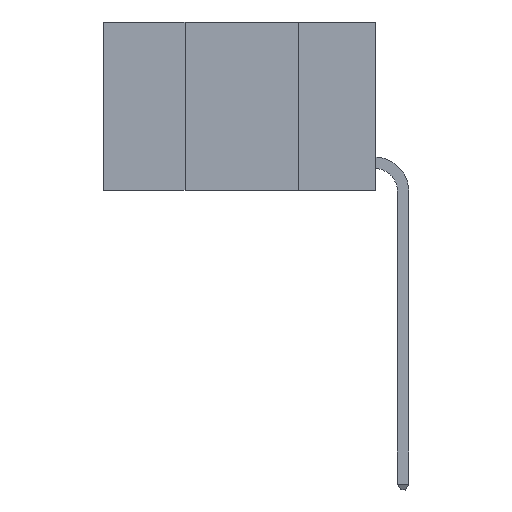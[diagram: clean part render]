
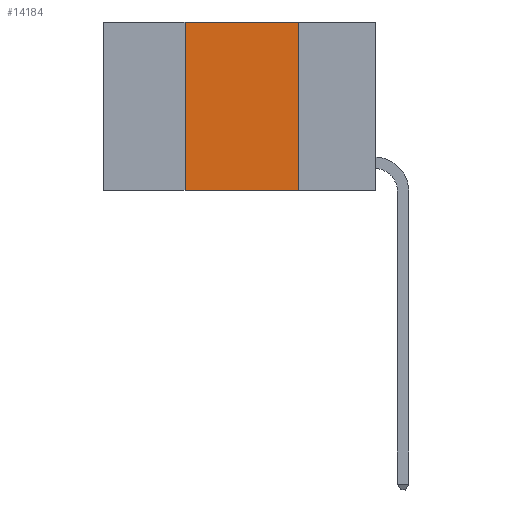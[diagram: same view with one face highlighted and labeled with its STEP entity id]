
A CAD part, left-side view. The second image highlights one B-rep face of the part: STEP entity #14184.
In plain terms, the highlighted planar face has unit normal (-1, 0, 0).
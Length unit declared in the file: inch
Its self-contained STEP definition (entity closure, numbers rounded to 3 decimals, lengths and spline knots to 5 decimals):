
#149 = CARTESIAN_POINT ( 'NONE',  ( 0., 0.17, -0.37 ) ) ;
#1687 = DIRECTION ( 'NONE',  ( 0., -1., 0. ) ) ;
#3434 = VERTEX_POINT ( 'NONE', #149 ) ;
#4382 = PLANE ( 'NONE',  #16585 ) ;
#5093 = EDGE_CURVE ( 'NONE', #20444, #3434, #11874, .T. ) ;
#5717 = LINE ( 'NONE', #27364, #12576 ) ;
#6720 = DIRECTION ( 'NONE',  ( 1., 0., 0. ) ) ;
#7209 = CARTESIAN_POINT ( 'NONE',  ( 0., 0.42, 0. ) ) ;
#8197 = EDGE_CURVE ( 'NONE', #22314, #3434, #5717, .T. ) ;
#8569 = EDGE_LOOP ( 'NONE', ( #14014, #21543, #13680, #11187 ) ) ;
#10779 = CARTESIAN_POINT ( 'NONE',  ( 0., 0.42, 0. ) ) ;
#11187 = ORIENTED_EDGE ( 'NONE', *, *, #5093, .T. ) ;
#11309 = FACE_OUTER_BOUND ( 'NONE', #8569, .T. ) ;
#11874 = LINE ( 'NONE', #22303, #29333 ) ;
#12576 = VECTOR ( 'NONE', #29629, 39.37008 ) ;
#12588 = CARTESIAN_POINT ( 'NONE',  ( 0., 0.42, -0.37 ) ) ;
#12648 = EDGE_CURVE ( 'NONE', #13353, #22314, #21616, .T. ) ;
#13353 = VERTEX_POINT ( 'NONE', #10779 ) ;
#13556 = CARTESIAN_POINT ( 'NONE',  ( 0., 0.6, 0. ) ) ;
#13680 = ORIENTED_EDGE ( 'NONE', *, *, #28636, .F. ) ;
#14014 = ORIENTED_EDGE ( 'NONE', *, *, #8197, .F. ) ;
#14184 = ADVANCED_FACE ( 'NONE', ( #11309 ), #4382, .F. ) ;
#15556 = VECTOR ( 'NONE', #26659, 39.37008 ) ;
#15734 = CARTESIAN_POINT ( 'NONE',  ( 0., 0.17, 0. ) ) ;
#16585 = AXIS2_PLACEMENT_3D ( 'NONE', #13556, #6720, #22734 ) ;
#20444 = VERTEX_POINT ( 'NONE', #12588 ) ;
#21543 = ORIENTED_EDGE ( 'NONE', *, *, #12648, .F. ) ;
#21616 = LINE ( 'NONE', #28844, #15556 ) ;
#22303 = CARTESIAN_POINT ( 'NONE',  ( 0., 0.6, -0.37 ) ) ;
#22314 = VERTEX_POINT ( 'NONE', #15734 ) ;
#22734 = DIRECTION ( 'NONE',  ( 0., 0., -1. ) ) ;
#25398 = DIRECTION ( 'NONE',  ( 0., 0., 1. ) ) ;
#26659 = DIRECTION ( 'NONE',  ( 0., -1., 0. ) ) ;
#27364 = CARTESIAN_POINT ( 'NONE',  ( 0., 0.17, 0. ) ) ;
#28503 = LINE ( 'NONE', #7209, #29230 ) ;
#28636 = EDGE_CURVE ( 'NONE', #20444, #13353, #28503, .T. ) ;
#28844 = CARTESIAN_POINT ( 'NONE',  ( 0., 0.6, 0. ) ) ;
#29230 = VECTOR ( 'NONE', #25398, 39.37008 ) ;
#29333 = VECTOR ( 'NONE', #1687, 39.37008 ) ;
#29629 = DIRECTION ( 'NONE',  ( 0., 0., -1. ) ) ;
